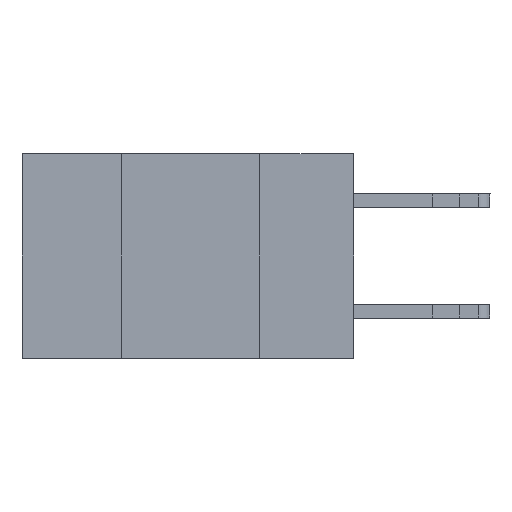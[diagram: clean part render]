
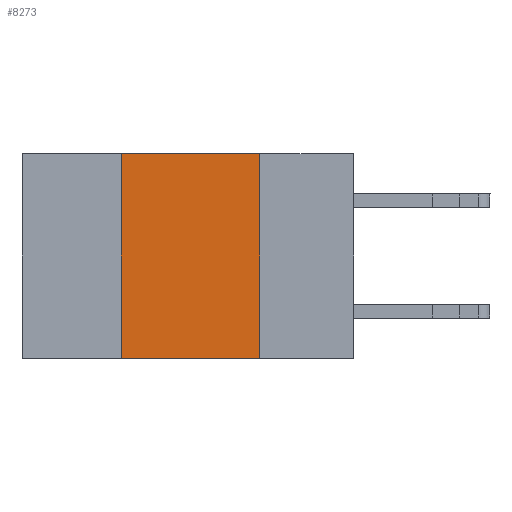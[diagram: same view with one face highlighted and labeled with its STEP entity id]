
A CAD part, left-side view. The second image highlights one B-rep face of the part: STEP entity #8273.
In plain terms, the highlighted planar face has unit normal (-1, 0, 0).
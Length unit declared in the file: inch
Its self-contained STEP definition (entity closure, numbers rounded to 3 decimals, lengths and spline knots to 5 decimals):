
#3333 = DIRECTION ( 'NONE',  ( 1., 0., 0. ) ) ;
#3453 = CARTESIAN_POINT ( 'NONE',  ( 0., 0.42, -0.37 ) ) ;
#4081 = CARTESIAN_POINT ( 'NONE',  ( 0., 0.42, 0. ) ) ;
#4720 = ORIENTED_EDGE ( 'NONE', *, *, #14338, .T. ) ;
#4869 = ORIENTED_EDGE ( 'NONE', *, *, #19942, .F. ) ;
#5820 = LINE ( 'NONE', #11256, #14333 ) ;
#6299 = DIRECTION ( 'NONE',  ( 0., -1., 0. ) ) ;
#7604 = CARTESIAN_POINT ( 'NONE',  ( 0., 0.6, 0. ) ) ;
#7805 = DIRECTION ( 'NONE',  ( 0., 0., 1. ) ) ;
#8273 = ADVANCED_FACE ( 'NONE', ( #10191 ), #16987, .F. ) ;
#8422 = DIRECTION ( 'NONE',  ( 0., 0., -1. ) ) ;
#8462 = EDGE_LOOP ( 'NONE', ( #15984, #4869, #9178, #4720 ) ) ;
#9178 = ORIENTED_EDGE ( 'NONE', *, *, #16253, .F. ) ;
#9440 = DIRECTION ( 'NONE',  ( 0., -1., 0. ) ) ;
#10133 = LINE ( 'NONE', #17127, #19880 ) ;
#10191 = FACE_OUTER_BOUND ( 'NONE', #8462, .T. ) ;
#10506 = VECTOR ( 'NONE', #9440, 39.37008 ) ;
#10665 = VERTEX_POINT ( 'NONE', #4081 ) ;
#11100 = VECTOR ( 'NONE', #6299, 39.37008 ) ;
#11256 = CARTESIAN_POINT ( 'NONE',  ( 0., 0.42, 0. ) ) ;
#12882 = AXIS2_PLACEMENT_3D ( 'NONE', #20535, #3333, #17296 ) ;
#14333 = VECTOR ( 'NONE', #7805, 39.37008 ) ;
#14338 = EDGE_CURVE ( 'NONE', #17974, #16335, #20184, .T. ) ;
#14703 = VERTEX_POINT ( 'NONE', #19566 ) ;
#14833 = LINE ( 'NONE', #7604, #10506 ) ;
#15022 = CARTESIAN_POINT ( 'NONE',  ( 0., 0.6, -0.37 ) ) ;
#15984 = ORIENTED_EDGE ( 'NONE', *, *, #22225, .F. ) ;
#16253 = EDGE_CURVE ( 'NONE', #17974, #10665, #5820, .T. ) ;
#16335 = VERTEX_POINT ( 'NONE', #21668 ) ;
#16987 = PLANE ( 'NONE',  #12882 ) ;
#17127 = CARTESIAN_POINT ( 'NONE',  ( 0., 0.17, 0. ) ) ;
#17296 = DIRECTION ( 'NONE',  ( 0., 0., -1. ) ) ;
#17974 = VERTEX_POINT ( 'NONE', #3453 ) ;
#19566 = CARTESIAN_POINT ( 'NONE',  ( 0., 0.17, 0. ) ) ;
#19880 = VECTOR ( 'NONE', #8422, 39.37008 ) ;
#19942 = EDGE_CURVE ( 'NONE', #10665, #14703, #14833, .T. ) ;
#20184 = LINE ( 'NONE', #15022, #11100 ) ;
#20535 = CARTESIAN_POINT ( 'NONE',  ( 0., 0.6, 0. ) ) ;
#21668 = CARTESIAN_POINT ( 'NONE',  ( 0., 0.17, -0.37 ) ) ;
#22225 = EDGE_CURVE ( 'NONE', #14703, #16335, #10133, .T. ) ;
